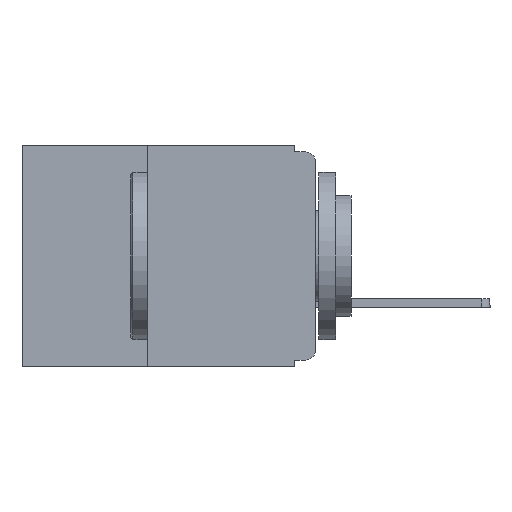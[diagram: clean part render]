
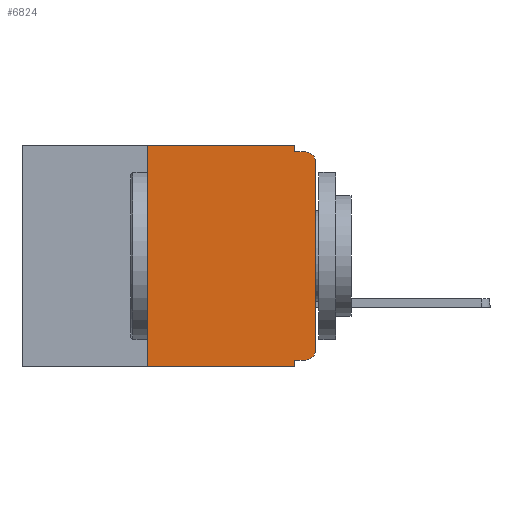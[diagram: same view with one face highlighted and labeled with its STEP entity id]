
A CAD part, left-side view. The second image highlights one B-rep face of the part: STEP entity #6824.
In plain terms, the highlighted planar face has unit normal (-1, 0, 0).
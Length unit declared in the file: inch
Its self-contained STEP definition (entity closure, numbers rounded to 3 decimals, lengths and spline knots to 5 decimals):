
#636 = ORIENTED_EDGE ( 'NONE', *, *, #12266, .F. ) ;
#687 = DIRECTION ( 'NONE',  ( 0., 0., -1. ) ) ;
#1217 = LINE ( 'NONE', #24285, #12878 ) ;
#1833 = DIRECTION ( 'NONE',  ( -1., 0., 0. ) ) ;
#2292 = CARTESIAN_POINT ( 'NONE',  ( 0., 0.031, 0. ) ) ;
#2679 = CARTESIAN_POINT ( 'NONE',  ( 0., 0.031, 0. ) ) ;
#3517 = DIRECTION ( 'NONE',  ( 0., -1., 0. ) ) ;
#3870 = CARTESIAN_POINT ( 'NONE',  ( 0., 0., 0. ) ) ;
#4804 = EDGE_CURVE ( 'NONE', #28994, #18375, #5727, .T. ) ;
#5727 = LINE ( 'NONE', #2292, #23293 ) ;
#5744 = LINE ( 'NONE', #16030, #13364 ) ;
#5917 = FACE_OUTER_BOUND ( 'NONE', #12592, .T. ) ;
#6600 = AXIS2_PLACEMENT_3D ( 'NONE', #26376, #25086, #24893 ) ;
#6824 = ADVANCED_FACE ( 'NONE', ( #5917 ), #25695, .F. ) ;
#6988 = EDGE_CURVE ( 'NONE', #22099, #21223, #19892, .T. ) ;
#8232 = AXIS2_PLACEMENT_3D ( 'NONE', #15697, #1833, #17972 ) ;
#8453 = EDGE_CURVE ( 'NONE', #21333, #21399, #29637, .T. ) ;
#8846 = DIRECTION ( 'NONE',  ( -1., 0., 0. ) ) ;
#9004 = CARTESIAN_POINT ( 'NONE',  ( 0., 0.031, -0.33 ) ) ;
#9165 = EDGE_CURVE ( 'NONE', #22099, #15666, #5744, .T. ) ;
#9664 = VECTOR ( 'NONE', #13561, 39.37008 ) ;
#10055 = LINE ( 'NONE', #17339, #22196 ) ;
#10392 = CIRCLE ( 'NONE', #8232, 0.015 ) ;
#10407 = LINE ( 'NONE', #9004, #9664 ) ;
#11207 = EDGE_CURVE ( 'NONE', #15692, #21333, #23951, .T. ) ;
#11273 = EDGE_CURVE ( 'NONE', #29553, #15692, #10392, .T. ) ;
#11464 = CARTESIAN_POINT ( 'NONE',  ( 0., 0.031, -0.32 ) ) ;
#11480 = CARTESIAN_POINT ( 'NONE',  ( 0., 0., -0.305 ) ) ;
#11845 = VECTOR ( 'NONE', #22258, 39.37008 ) ;
#12266 = EDGE_CURVE ( 'NONE', #21223, #28994, #1217, .T. ) ;
#12592 = EDGE_LOOP ( 'NONE', ( #20380, #27902, #24496, #18073, #636, #28960, #24988, #19782, #19958, #24059 ) ) ;
#12878 = VECTOR ( 'NONE', #26518, 39.37008 ) ;
#13364 = VECTOR ( 'NONE', #18310, 39.37008 ) ;
#13561 = DIRECTION ( 'NONE',  ( 0., 0., -1. ) ) ;
#13679 = CARTESIAN_POINT ( 'NONE',  ( 0., 0.031, -0.33 ) ) ;
#14105 = CARTESIAN_POINT ( 'NONE',  ( 0., 0.015, -0.32 ) ) ;
#15241 = CARTESIAN_POINT ( 'NONE',  ( 0., 0.25, 0. ) ) ;
#15625 = CARTESIAN_POINT ( 'NONE',  ( 0., 0., -0.025 ) ) ;
#15666 = VERTEX_POINT ( 'NONE', #13679 ) ;
#15692 = VERTEX_POINT ( 'NONE', #11480 ) ;
#15697 = CARTESIAN_POINT ( 'NONE',  ( 0., 0.015, -0.305 ) ) ;
#16030 = CARTESIAN_POINT ( 'NONE',  ( 0., 0.437, -0.33 ) ) ;
#17339 = CARTESIAN_POINT ( 'NONE',  ( 0., 0., -0.01 ) ) ;
#17919 = CARTESIAN_POINT ( 'NONE',  ( 0., 0.25, -0.33 ) ) ;
#17972 = DIRECTION ( 'NONE',  ( 0., 0., -1. ) ) ;
#18073 = ORIENTED_EDGE ( 'NONE', *, *, #4804, .F. ) ;
#18273 = CARTESIAN_POINT ( 'NONE',  ( 0., 0., -0.32 ) ) ;
#18310 = DIRECTION ( 'NONE',  ( 0., -1., 0. ) ) ;
#18375 = VERTEX_POINT ( 'NONE', #27277 ) ;
#19198 = VECTOR ( 'NONE', #21183, 39.37008 ) ;
#19782 = ORIENTED_EDGE ( 'NONE', *, *, #20897, .F. ) ;
#19892 = LINE ( 'NONE', #21150, #19198 ) ;
#19958 = ORIENTED_EDGE ( 'NONE', *, *, #27611, .F. ) ;
#20380 = ORIENTED_EDGE ( 'NONE', *, *, #11207, .T. ) ;
#20635 = EDGE_CURVE ( 'NONE', #18375, #21399, #10055, .T. ) ;
#20897 = EDGE_CURVE ( 'NONE', #23483, #15666, #10407, .T. ) ;
#20964 = LINE ( 'NONE', #18273, #26266 ) ;
#21150 = CARTESIAN_POINT ( 'NONE',  ( 0., 0.25, -0.33 ) ) ;
#21183 = DIRECTION ( 'NONE',  ( 0., 0., 1. ) ) ;
#21223 = VERTEX_POINT ( 'NONE', #15241 ) ;
#21333 = VERTEX_POINT ( 'NONE', #15625 ) ;
#21399 = VERTEX_POINT ( 'NONE', #25040 ) ;
#22099 = VERTEX_POINT ( 'NONE', #17919 ) ;
#22196 = VECTOR ( 'NONE', #3517, 39.37008 ) ;
#22258 = DIRECTION ( 'NONE',  ( 0., 0., 1. ) ) ;
#22538 = CARTESIAN_POINT ( 'NONE',  ( 0., 0.015, -0.025 ) ) ;
#23293 = VECTOR ( 'NONE', #687, 39.37008 ) ;
#23483 = VERTEX_POINT ( 'NONE', #11464 ) ;
#23951 = LINE ( 'NONE', #3870, #11845 ) ;
#24059 = ORIENTED_EDGE ( 'NONE', *, *, #11273, .T. ) ;
#24285 = CARTESIAN_POINT ( 'NONE',  ( 0., 0.437, 0. ) ) ;
#24496 = ORIENTED_EDGE ( 'NONE', *, *, #20635, .F. ) ;
#24800 = DIRECTION ( 'NONE',  ( 0., 0., -1. ) ) ;
#24893 = DIRECTION ( 'NONE',  ( 0., 0., -1. ) ) ;
#24988 = ORIENTED_EDGE ( 'NONE', *, *, #9165, .T. ) ;
#25040 = CARTESIAN_POINT ( 'NONE',  ( 0., 0.015, -0.01 ) ) ;
#25086 = DIRECTION ( 'NONE',  ( 1., 0., 0. ) ) ;
#25198 = AXIS2_PLACEMENT_3D ( 'NONE', #22538, #8846, #24800 ) ;
#25695 = PLANE ( 'NONE',  #6600 ) ;
#26266 = VECTOR ( 'NONE', #27264, 39.37008 ) ;
#26376 = CARTESIAN_POINT ( 'NONE',  ( 0., 0.437, 0. ) ) ;
#26518 = DIRECTION ( 'NONE',  ( 0., -1., 0. ) ) ;
#27264 = DIRECTION ( 'NONE',  ( 0., 1., 0. ) ) ;
#27277 = CARTESIAN_POINT ( 'NONE',  ( 0., 0.031, -0.01 ) ) ;
#27611 = EDGE_CURVE ( 'NONE', #29553, #23483, #20964, .T. ) ;
#27902 = ORIENTED_EDGE ( 'NONE', *, *, #8453, .T. ) ;
#28960 = ORIENTED_EDGE ( 'NONE', *, *, #6988, .F. ) ;
#28994 = VERTEX_POINT ( 'NONE', #2679 ) ;
#29553 = VERTEX_POINT ( 'NONE', #14105 ) ;
#29637 = CIRCLE ( 'NONE', #25198, 0.015 ) ;
